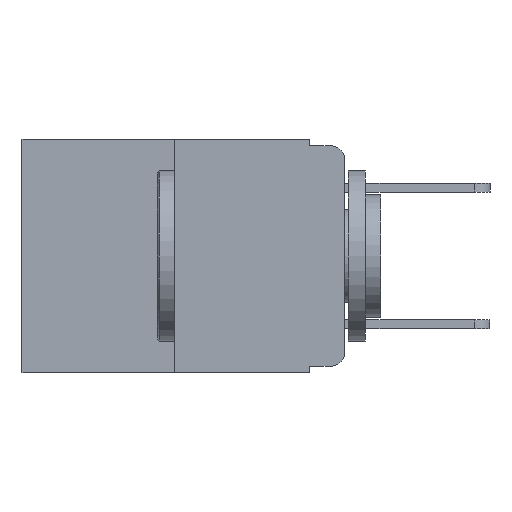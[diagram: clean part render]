
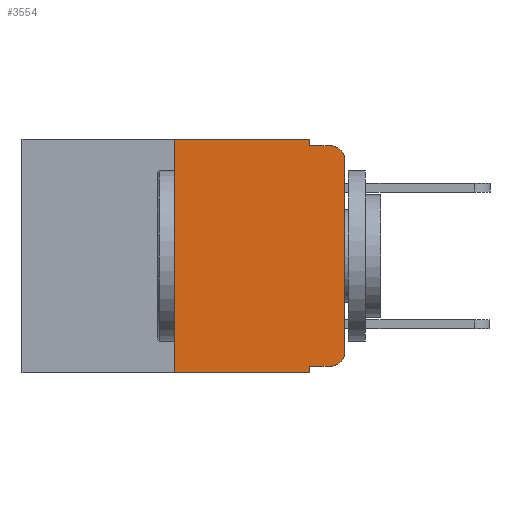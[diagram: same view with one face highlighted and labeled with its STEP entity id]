
A CAD part, left-side view. The second image highlights one B-rep face of the part: STEP entity #3554.
In plain terms, the highlighted planar face has unit normal (-1, 0, 0).
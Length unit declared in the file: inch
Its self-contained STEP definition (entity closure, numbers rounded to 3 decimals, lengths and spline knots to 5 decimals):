
#4 = PLANE ( 'NONE',  #3964 ) ;
#84 = VERTEX_POINT ( 'NONE', #9952 ) ;
#134 = VERTEX_POINT ( 'NONE', #9566 ) ;
#214 = CARTESIAN_POINT ( 'NONE',  ( 0., 0.02, -0.01 ) ) ;
#230 = CARTESIAN_POINT ( 'NONE',  ( 0., 0.051, -0.01 ) ) ;
#300 = CARTESIAN_POINT ( 'NONE',  ( 0., 0.473, -0.343 ) ) ;
#401 = EDGE_CURVE ( 'NONE', #7130, #4808, #9981, .T. ) ;
#874 = VERTEX_POINT ( 'NONE', #214 ) ;
#1087 = EDGE_CURVE ( 'NONE', #134, #7253, #8332, .T. ) ;
#1114 = CARTESIAN_POINT ( 'NONE',  ( 0., 0.051, -0.333 ) ) ;
#1205 = DIRECTION ( 'NONE',  ( 0., 0., 1. ) ) ;
#1399 = DIRECTION ( 'NONE',  ( 1., 0., 0. ) ) ;
#1437 = EDGE_CURVE ( 'NONE', #84, #2412, #3471, .T. ) ;
#1449 = CARTESIAN_POINT ( 'NONE',  ( 0., 0., -0.313 ) ) ;
#1596 = CARTESIAN_POINT ( 'NONE',  ( 0., 0.473, 0. ) ) ;
#2257 = ORIENTED_EDGE ( 'NONE', *, *, #10349, .T. ) ;
#2261 = VECTOR ( 'NONE', #9994, 39.37008 ) ;
#2366 = ORIENTED_EDGE ( 'NONE', *, *, #7882, .T. ) ;
#2412 = VERTEX_POINT ( 'NONE', #7567 ) ;
#2507 = ORIENTED_EDGE ( 'NONE', *, *, #8083, .F. ) ;
#2573 = DIRECTION ( 'NONE',  ( 0., -1., 0. ) ) ;
#2727 = ORIENTED_EDGE ( 'NONE', *, *, #7465, .F. ) ;
#2813 = CARTESIAN_POINT ( 'NONE',  ( 0., 0.02, -0.313 ) ) ;
#2855 = DIRECTION ( 'NONE',  ( 0., 0., -1. ) ) ;
#2970 = DIRECTION ( 'NONE',  ( 0., -1., 0. ) ) ;
#3035 = VECTOR ( 'NONE', #1205, 39.37008 ) ;
#3053 = CARTESIAN_POINT ( 'NONE',  ( 0., 0.051, -0.01 ) ) ;
#3137 = CARTESIAN_POINT ( 'NONE',  ( 0., 0., -0.03 ) ) ;
#3172 = ORIENTED_EDGE ( 'NONE', *, *, #1087, .F. ) ;
#3310 = ORIENTED_EDGE ( 'NONE', *, *, #7024, .F. ) ;
#3318 = LINE ( 'NONE', #9369, #3035 ) ;
#3471 = LINE ( 'NONE', #1114, #9507 ) ;
#3513 = DIRECTION ( 'NONE',  ( 0., 0., -1. ) ) ;
#3554 = ADVANCED_FACE ( 'NONE', ( #5428 ), #4, .F. ) ;
#3580 = ORIENTED_EDGE ( 'NONE', *, *, #401, .T. ) ;
#3722 = DIRECTION ( 'NONE',  ( 0., 0., -1. ) ) ;
#3776 = CARTESIAN_POINT ( 'NONE',  ( 0., 0.051, -0.343 ) ) ;
#3819 = DIRECTION ( 'NONE',  ( 0., -1., 0. ) ) ;
#3865 = ORIENTED_EDGE ( 'NONE', *, *, #7292, .F. ) ;
#3964 = AXIS2_PLACEMENT_3D ( 'NONE', #1596, #1399, #9809 ) ;
#3999 = ORIENTED_EDGE ( 'NONE', *, *, #1437, .T. ) ;
#4568 = DIRECTION ( 'NONE',  ( 0., 0., 1. ) ) ;
#4583 = VECTOR ( 'NONE', #3513, 39.37008 ) ;
#4646 = ORIENTED_EDGE ( 'NONE', *, *, #7416, .T. ) ;
#4808 = VERTEX_POINT ( 'NONE', #3776 ) ;
#4847 = LINE ( 'NONE', #9779, #4583 ) ;
#4900 = VERTEX_POINT ( 'NONE', #3053 ) ;
#4922 = CARTESIAN_POINT ( 'NONE',  ( 0., 0.473, 0. ) ) ;
#4945 = VERTEX_POINT ( 'NONE', #1449 ) ;
#5224 = CARTESIAN_POINT ( 'NONE',  ( 0., 0.02, -0.03 ) ) ;
#5272 = EDGE_LOOP ( 'NONE', ( #2257, #2366, #2507, #2727, #3172, #3310, #3580, #3865, #3999, #4646 ) ) ;
#5368 = CARTESIAN_POINT ( 'NONE',  ( 0., 0.25, 0. ) ) ;
#5428 = FACE_OUTER_BOUND ( 'NONE', #5272, .T. ) ;
#5489 = LINE ( 'NONE', #5368, #9315 ) ;
#5717 = CIRCLE ( 'NONE', #9733, 0.02 ) ;
#5795 = AXIS2_PLACEMENT_3D ( 'NONE', #5224, #10482, #5996 ) ;
#5958 = VECTOR ( 'NONE', #3819, 39.37008 ) ;
#5996 = DIRECTION ( 'NONE',  ( 0., 0., -1. ) ) ;
#6331 = VECTOR ( 'NONE', #2573, 39.37008 ) ;
#6631 = VERTEX_POINT ( 'NONE', #3137 ) ;
#7024 = EDGE_CURVE ( 'NONE', #7130, #134, #5489, .T. ) ;
#7130 = VERTEX_POINT ( 'NONE', #8058 ) ;
#7253 = VERTEX_POINT ( 'NONE', #10461 ) ;
#7292 = EDGE_CURVE ( 'NONE', #84, #4808, #4847, .T. ) ;
#7416 = EDGE_CURVE ( 'NONE', #2412, #4945, #5717, .T. ) ;
#7465 = EDGE_CURVE ( 'NONE', #7253, #4900, #9307, .T. ) ;
#7567 = CARTESIAN_POINT ( 'NONE',  ( 0., 0.02, -0.333 ) ) ;
#7882 = EDGE_CURVE ( 'NONE', #6631, #874, #9300, .T. ) ;
#8058 = CARTESIAN_POINT ( 'NONE',  ( 0., 0.25, -0.343 ) ) ;
#8083 = EDGE_CURVE ( 'NONE', #4900, #874, #8715, .T. ) ;
#8332 = LINE ( 'NONE', #4922, #6331 ) ;
#8465 = DIRECTION ( 'NONE',  ( -1., 0., 0. ) ) ;
#8715 = LINE ( 'NONE', #230, #2261 ) ;
#9071 = VECTOR ( 'NONE', #2855, 39.37008 ) ;
#9249 = CARTESIAN_POINT ( 'NONE',  ( 0., 0.051, 0. ) ) ;
#9300 = CIRCLE ( 'NONE', #5795, 0.02 ) ;
#9307 = LINE ( 'NONE', #9249, #9071 ) ;
#9315 = VECTOR ( 'NONE', #4568, 39.37008 ) ;
#9369 = CARTESIAN_POINT ( 'NONE',  ( 0., 0., 0. ) ) ;
#9507 = VECTOR ( 'NONE', #2970, 39.37008 ) ;
#9566 = CARTESIAN_POINT ( 'NONE',  ( 0., 0.25, 0. ) ) ;
#9733 = AXIS2_PLACEMENT_3D ( 'NONE', #2813, #8465, #3722 ) ;
#9779 = CARTESIAN_POINT ( 'NONE',  ( 0., 0.051, 0. ) ) ;
#9809 = DIRECTION ( 'NONE',  ( 0., 0., -1. ) ) ;
#9952 = CARTESIAN_POINT ( 'NONE',  ( 0., 0.051, -0.333 ) ) ;
#9981 = LINE ( 'NONE', #300, #5958 ) ;
#9994 = DIRECTION ( 'NONE',  ( 0., -1., 0. ) ) ;
#10349 = EDGE_CURVE ( 'NONE', #4945, #6631, #3318, .T. ) ;
#10461 = CARTESIAN_POINT ( 'NONE',  ( 0., 0.051, 0. ) ) ;
#10482 = DIRECTION ( 'NONE',  ( -1., 0., 0. ) ) ;
